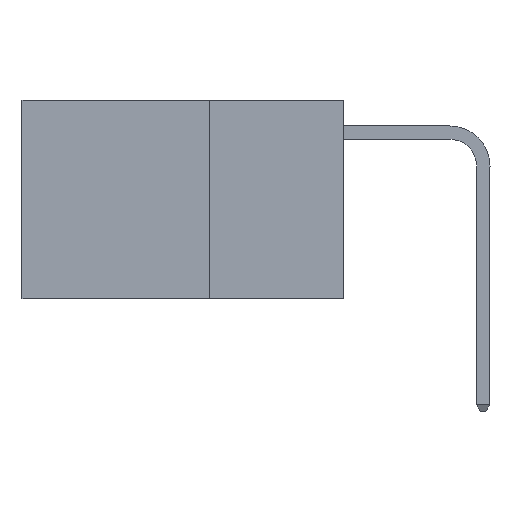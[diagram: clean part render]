
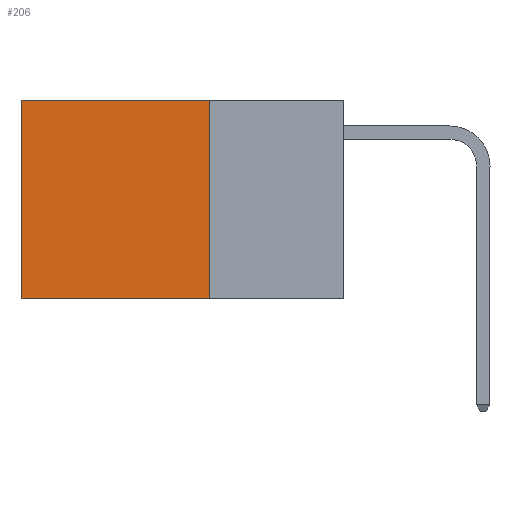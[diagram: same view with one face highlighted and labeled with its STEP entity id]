
A CAD part, left-side view. The second image highlights one B-rep face of the part: STEP entity #206.
In plain terms, the highlighted planar face has unit normal (-1, 0, 0).
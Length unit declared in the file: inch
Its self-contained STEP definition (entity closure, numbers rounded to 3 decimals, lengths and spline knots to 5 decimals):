
#206 = ADVANCED_FACE ( 'NONE', ( #3291 ), #2994, .F. ) ;
#256 = ORIENTED_EDGE ( 'NONE', *, *, #3522, .T. ) ;
#360 = CARTESIAN_POINT ( 'NONE',  ( 0.2625, 0.6, -0.37 ) ) ;
#1295 = DIRECTION ( 'NONE',  ( 0., 0., -1. ) ) ;
#1603 = DIRECTION ( 'NONE',  ( 1., 0., 0. ) ) ;
#1929 = VERTEX_POINT ( 'NONE', #4506 ) ;
#2428 = AXIS2_PLACEMENT_3D ( 'NONE', #13480, #1603, #14127 ) ;
#2741 = ORIENTED_EDGE ( 'NONE', *, *, #12320, .F. ) ;
#2994 = PLANE ( 'NONE',  #2428 ) ;
#3291 = FACE_OUTER_BOUND ( 'NONE', #12568, .T. ) ;
#3522 = EDGE_CURVE ( 'NONE', #5940, #8554, #12887, .T. ) ;
#3678 = ORIENTED_EDGE ( 'NONE', *, *, #6529, .F. ) ;
#3850 = VECTOR ( 'NONE', #1295, 39.37008 ) ;
#4407 = VECTOR ( 'NONE', #14044, 39.37008 ) ;
#4506 = CARTESIAN_POINT ( 'NONE',  ( 0.2625, 0.25, -0.37 ) ) ;
#5070 = LINE ( 'NONE', #6186, #5152 ) ;
#5152 = VECTOR ( 'NONE', #6174, 39.37008 ) ;
#5940 = VERTEX_POINT ( 'NONE', #10407 ) ;
#6174 = DIRECTION ( 'NONE',  ( 0., 0., -1. ) ) ;
#6186 = CARTESIAN_POINT ( 'NONE',  ( 0.2625, 0.25, 0. ) ) ;
#6529 = EDGE_CURVE ( 'NONE', #5940, #1929, #5070, .T. ) ;
#8115 = DIRECTION ( 'NONE',  ( 0., 1., 0. ) ) ;
#8420 = CARTESIAN_POINT ( 'NONE',  ( 0.2625, 0.25, 0. ) ) ;
#8554 = VERTEX_POINT ( 'NONE', #12175 ) ;
#9078 = CARTESIAN_POINT ( 'NONE',  ( 0.2625, 0.6, 0. ) ) ;
#9739 = LINE ( 'NONE', #9078, #3850 ) ;
#10292 = VERTEX_POINT ( 'NONE', #360 ) ;
#10407 = CARTESIAN_POINT ( 'NONE',  ( 0.2625, 0.25, 0. ) ) ;
#10613 = LINE ( 'NONE', #13015, #4407 ) ;
#12175 = CARTESIAN_POINT ( 'NONE',  ( 0.2625, 0.6, 0. ) ) ;
#12320 = EDGE_CURVE ( 'NONE', #1929, #10292, #10613, .T. ) ;
#12487 = EDGE_CURVE ( 'NONE', #8554, #10292, #9739, .T. ) ;
#12536 = ORIENTED_EDGE ( 'NONE', *, *, #12487, .T. ) ;
#12568 = EDGE_LOOP ( 'NONE', ( #12536, #2741, #3678, #256 ) ) ;
#12841 = VECTOR ( 'NONE', #8115, 39.37008 ) ;
#12887 = LINE ( 'NONE', #8420, #12841 ) ;
#13015 = CARTESIAN_POINT ( 'NONE',  ( 0.2625, 0.25, -0.37 ) ) ;
#13480 = CARTESIAN_POINT ( 'NONE',  ( 0.2625, 0.25, 0. ) ) ;
#14044 = DIRECTION ( 'NONE',  ( 0., 1., 0. ) ) ;
#14127 = DIRECTION ( 'NONE',  ( 0., 0., -1. ) ) ;
